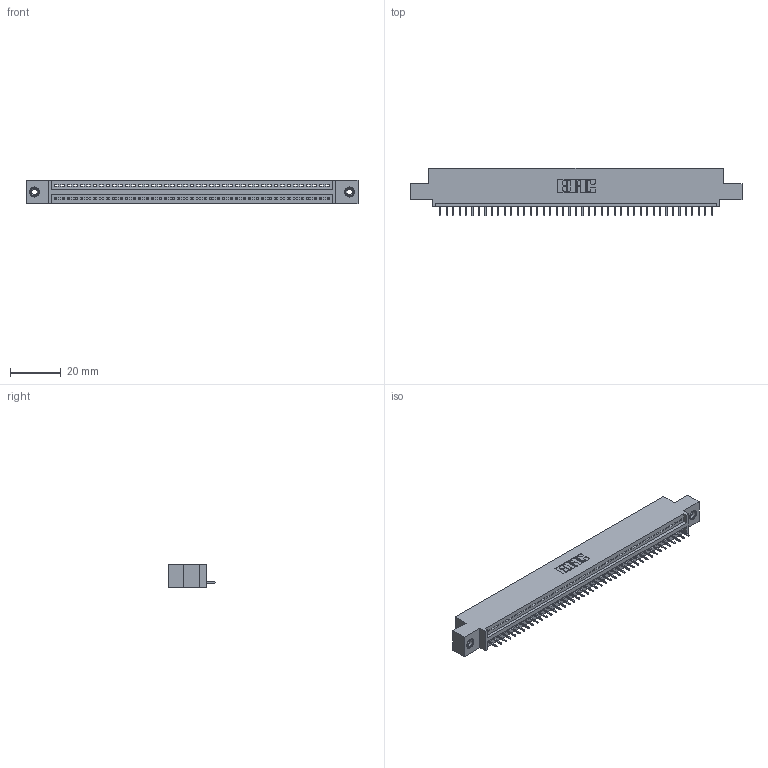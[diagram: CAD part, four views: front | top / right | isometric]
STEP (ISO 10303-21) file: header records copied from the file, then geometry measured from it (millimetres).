
FILE_DESCRIPTION (( 'STEP AP203' ), '1' );
FILE_NAME ('345-043-525-408.STEP', '2020-09-19T21:36:27', ( '' ), ( '' ), 'SwSTEP 2.0', 'SolidWorks 2020', '' );
FILE_SCHEMA (( 'CONFIG_CONTROL_DESIGN' ));
Length unit declared in the file: inch
Products named in the file (4): 345-250-001_345-250-003-102; 345 Part_0.110 Offset - 0.156 Dia-TI; 345-292-001_345-293-125; 345-043-525-408
Assembly tree (46 placements, depth 2):
  345-043-525-408
    345 Part_0.110 Offset - 0.156 Dia-TI
    345-292-001_345-293-125  x43
    345-250-001_345-250-003-102  x2
Bounding box: 130.43 x 18.72 x 9.4 mm (x, y, z)
Volume: 12141 mm3; surface area: 15663.5 mm2
Topology: 46 solids, 46 shells, 2856 faces, 8229 edges, 5306 vertices
Faces by surface type: plane 2094, cylinder 746, cone 12, torus 4
Entity records: 33620 total; most frequent: CARTESIAN_POINT 5804, ORIENTED_EDGE 5774, DIRECTION 5095, EDGE_CURVE 2887, LINE 2567, VECTOR 2567, VERTEX_POINT 1916, AXIS2_PLACEMENT_3D 1264
